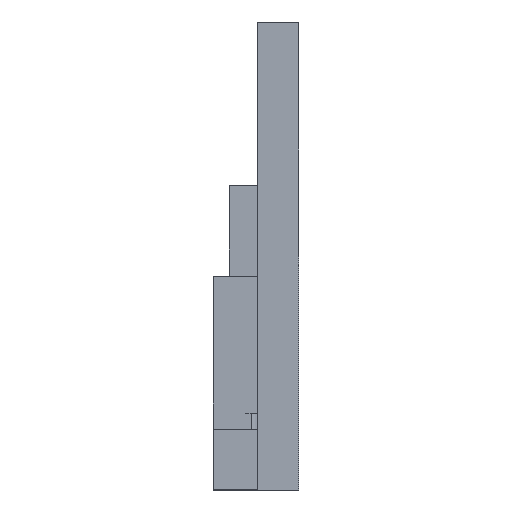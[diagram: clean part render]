
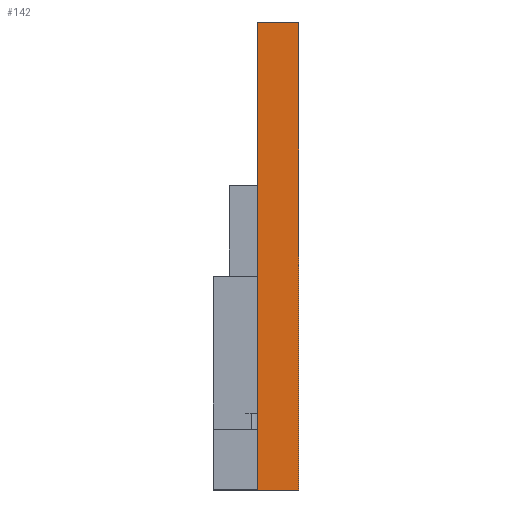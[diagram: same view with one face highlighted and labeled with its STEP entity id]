
A CAD part, left-side view. The second image highlights one B-rep face of the part: STEP entity #142.
In plain terms, the highlighted planar face has unit normal (-1, 0, 0).
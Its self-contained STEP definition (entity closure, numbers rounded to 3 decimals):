
#74 = VERTEX_POINT ( 'NONE', #630 ) ;
#86 = EDGE_CURVE ( 'NONE', #1959, #1900, #1049, .T. ) ;
#142 = ADVANCED_FACE ( 'NONE', ( #1789 ), #1880, .F. ) ;
#187 = VECTOR ( 'NONE', #348, 1000. ) ;
#195 = AXIS2_PLACEMENT_3D ( 'NONE', #1105, #1263, #613 ) ;
#348 = DIRECTION ( 'NONE',  ( 0., 0., 1. ) ) ;
#371 = VECTOR ( 'NONE', #395, 1000. ) ;
#395 = DIRECTION ( 'NONE',  ( 0., 0., 1. ) ) ;
#418 = LINE ( 'NONE', #1026, #371 ) ;
#481 = EDGE_CURVE ( 'NONE', #74, #526, #418, .T. ) ;
#526 = VERTEX_POINT ( 'NONE', #1797 ) ;
#596 = CARTESIAN_POINT ( 'NONE',  ( -93.25, 6.4, -36.5 ) ) ;
#613 = DIRECTION ( 'NONE',  ( 0., 0., -1. ) ) ;
#630 = CARTESIAN_POINT ( 'NONE',  ( -93.25, 0., -36.5 ) ) ;
#1026 = CARTESIAN_POINT ( 'NONE',  ( -93.25, 0., 36.5 ) ) ;
#1049 = LINE ( 'NONE', #1269, #187 ) ;
#1053 = CARTESIAN_POINT ( 'NONE',  ( -93.25, 6.4, 36.5 ) ) ;
#1079 = ORIENTED_EDGE ( 'NONE', *, *, #1835, .F. ) ;
#1105 = CARTESIAN_POINT ( 'NONE',  ( -93.25, 6.4, 36.5 ) ) ;
#1124 = ORIENTED_EDGE ( 'NONE', *, *, #86, .F. ) ;
#1127 = EDGE_LOOP ( 'NONE', ( #1400, #1079, #1124, #1336 ) ) ;
#1205 = DIRECTION ( 'NONE',  ( 0., -1., 0. ) ) ;
#1263 = DIRECTION ( 'NONE',  ( 1., 0., 0. ) ) ;
#1269 = CARTESIAN_POINT ( 'NONE',  ( -93.25, 6.4, 36.5 ) ) ;
#1336 = ORIENTED_EDGE ( 'NONE', *, *, #1776, .T. ) ;
#1351 = LINE ( 'NONE', #596, #1937 ) ;
#1359 = DIRECTION ( 'NONE',  ( 0., -1., 0. ) ) ;
#1400 = ORIENTED_EDGE ( 'NONE', *, *, #481, .T. ) ;
#1545 = LINE ( 'NONE', #1053, #1571 ) ;
#1571 = VECTOR ( 'NONE', #1359, 1000. ) ;
#1604 = CARTESIAN_POINT ( 'NONE',  ( -93.25, 6.4, 36.5 ) ) ;
#1775 = CARTESIAN_POINT ( 'NONE',  ( -93.25, 6.4, -36.5 ) ) ;
#1776 = EDGE_CURVE ( 'NONE', #1959, #74, #1351, .T. ) ;
#1789 = FACE_OUTER_BOUND ( 'NONE', #1127, .T. ) ;
#1797 = CARTESIAN_POINT ( 'NONE',  ( -93.25, 0., 36.5 ) ) ;
#1835 = EDGE_CURVE ( 'NONE', #1900, #526, #1545, .T. ) ;
#1880 = PLANE ( 'NONE',  #195 ) ;
#1900 = VERTEX_POINT ( 'NONE', #1604 ) ;
#1937 = VECTOR ( 'NONE', #1205, 1000. ) ;
#1959 = VERTEX_POINT ( 'NONE', #1775 ) ;
